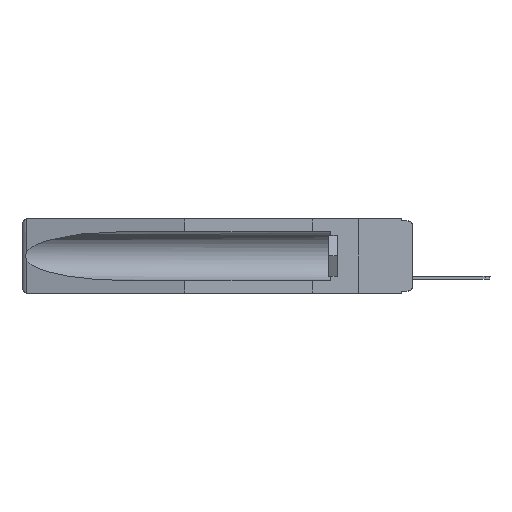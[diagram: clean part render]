
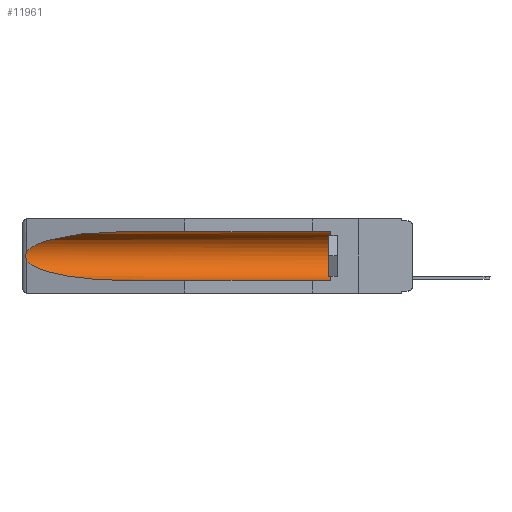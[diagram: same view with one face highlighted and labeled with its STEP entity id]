
A CAD part, left-side view. The second image highlights one B-rep face of the part: STEP entity #11961.
In plain terms, the highlighted cylindrical face has radius 2.857 mm (diameter 5.715 mm), a partial arc.
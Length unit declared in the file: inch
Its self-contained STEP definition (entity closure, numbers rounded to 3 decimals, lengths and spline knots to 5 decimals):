
#261 = DIRECTION ( 'NONE',  ( 0., -1., 0. ) ) ;
#290 = ORIENTED_EDGE ( 'NONE', *, *, #14992, .T. ) ;
#526 = CARTESIAN_POINT ( 'NONE',  ( 0.2673, 1.5327, -0.16383 ) ) ;
#824 = CARTESIAN_POINT ( 'NONE',  ( 0.155, 1.07973, -0.059 ) ) ;
#921 = CARTESIAN_POINT ( 'NONE',  ( 0.26597, 1.5296, -0.19026 ) ) ;
#1210 = CARTESIAN_POINT ( 'NONE',  ( 0.26537, 1.52718, -0.19328 ) ) ;
#1668 = CARTESIAN_POINT ( 'NONE',  ( 0.26537, 1.52718, -0.14972 ) ) ;
#1896 = CARTESIAN_POINT ( 'NONE',  ( 0.2675, 1.53308, -0.17534 ) ) ;
#1996 = VERTEX_POINT ( 'NONE', #824 ) ;
#2424 = CARTESIAN_POINT ( 'NONE',  ( 0.26537, 1.52718, -0.19328 ) ) ;
#3214 = CARTESIAN_POINT ( 'NONE',  ( 0.25451, 1.48313, -0.09465 ) ) ;
#3431 = LINE ( 'NONE', #4600, #3913 ) ;
#3781 = CARTESIAN_POINT ( 'NONE',  ( 0.2673, 1.53269, -0.17917 ) ) ;
#3913 = VECTOR ( 'NONE', #6248, 39.37008 ) ;
#4562 = CARTESIAN_POINT ( 'NONE',  ( 0.155, 0.126, -0.059 ) ) ;
#4600 = CARTESIAN_POINT ( 'NONE',  ( 0.155, -0.30754, -0.059 ) ) ;
#4889 = CARTESIAN_POINT ( 'NONE',  ( 0.155, 0.126, -0.284 ) ) ;
#4952 = DIRECTION ( 'NONE',  ( 0., 0., 1. ) ) ;
#5081 = CARTESIAN_POINT ( 'NONE',  ( 0.155, -0.30754, -0.284 ) ) ;
#5817 = ORIENTED_EDGE ( 'NONE', *, *, #17352, .T. ) ;
#5830 = CARTESIAN_POINT ( 'NONE',  ( 0.21114, 1.30732, -0.284 ) ) ;
#6248 = DIRECTION ( 'NONE',  ( 0., 1., 0. ) ) ;
#6476 = CARTESIAN_POINT ( 'NONE',  ( 0.155, 1.07973, -0.284 ) ) ;
#6992 = ORIENTED_EDGE ( 'NONE', *, *, #13037, .T. ) ;
#7486 = VECTOR ( 'NONE', #17554, 39.37008 ) ;
#7591 = B_SPLINE_CURVE_WITH_KNOTS ( 'NONE', 3,
 ( #15887, #8298, #17680, #526, #14537, #1896, #3781, #11750, #921, #2424 ),
 .UNSPECIFIED., .F., .F.,
 ( 4, 2, 2, 2, 4 ),
 ( 0., 0.00029, 0.00058, 0.00087, 0.00117 ),
 .UNSPECIFIED. ) ;
#7593 = CARTESIAN_POINT ( 'NONE',  ( 0.155, 1.07973, -0.284 ) ) ;
#8298 = CARTESIAN_POINT ( 'NONE',  ( 0.26597, 1.52961, -0.15275 ) ) ;
#8745 = FACE_OUTER_BOUND ( 'NONE', #11232, .T. ) ;
#8973 = LINE ( 'NONE', #5081, #7486 ) ;
#9035 = ORIENTED_EDGE ( 'NONE', *, *, #14960, .F. ) ;
#9303 = VERTEX_POINT ( 'NONE', #6476 ) ;
#9597 = CARTESIAN_POINT ( 'NONE',  ( 0.155, 0.126, -0.1715 ) ) ;
#9755 = CARTESIAN_POINT ( 'NONE',  ( 0.26537, 1.52718, -0.14972 ) ) ;
#9760 = ORIENTED_EDGE ( 'NONE', *, *, #15395, .T. ) ;
#9935 = EDGE_CURVE ( 'NONE', #19535, #9303, #16304, .T. ) ;
#10086 = VERTEX_POINT ( 'NONE', #4889 ) ;
#10410 = DIRECTION ( 'NONE',  ( 0., 1., 0. ) ) ;
#10870 = ORIENTED_EDGE ( 'NONE', *, *, #9935, .T. ) ;
#11232 = EDGE_LOOP ( 'NONE', ( #9760, #290, #10870, #9035, #6992, #5817 ) ) ;
#11750 = CARTESIAN_POINT ( 'NONE',  ( 0.26655, 1.53094, -0.18657 ) ) ;
#11961 = ADVANCED_FACE ( 'NONE', ( #8745 ), #18419, .F. ) ;
#12300 = CARTESIAN_POINT ( 'NONE',  ( 0.25451, 1.48313, -0.24835 ) ) ;
#12471 =( BOUNDED_CURVE ( )  B_SPLINE_CURVE ( 3, ( #13891, #20075, #3214, #1668 ),
 .UNSPECIFIED., .F., .T. ) 
 B_SPLINE_CURVE_WITH_KNOTS ( ( 4, 4 ),
 ( 4.71239, 6.08839 ),
 .UNSPECIFIED. ) 
 CURVE ( )  GEOMETRIC_REPRESENTATION_ITEM ( )  RATIONAL_B_SPLINE_CURVE ( ( 1., 0.848, 0.848, 1. ) ) 
 REPRESENTATION_ITEM ( '' )  );
#13037 = EDGE_CURVE ( 'NONE', #10086, #19279, #15030, .T. ) ;
#13251 = DIRECTION ( 'NONE',  ( 0., 0., 1. ) ) ;
#13891 = CARTESIAN_POINT ( 'NONE',  ( 0.155, 1.07973, -0.059 ) ) ;
#14537 = CARTESIAN_POINT ( 'NONE',  ( 0.2675, 1.53308, -0.16763 ) ) ;
#14960 = EDGE_CURVE ( 'NONE', #10086, #9303, #8973, .T. ) ;
#14992 = EDGE_CURVE ( 'NONE', #17053, #19535, #7591, .T. ) ;
#15030 = CIRCLE ( 'NONE', #15631, 0.1125 ) ;
#15395 = EDGE_CURVE ( 'NONE', #1996, #17053, #12471, .T. ) ;
#15631 = AXIS2_PLACEMENT_3D ( 'NONE', #9597, #261, #4952 ) ;
#15887 = CARTESIAN_POINT ( 'NONE',  ( 0.26537, 1.52718, -0.14972 ) ) ;
#16176 = CARTESIAN_POINT ( 'NONE',  ( 0.26537, 1.52718, -0.19328 ) ) ;
#16304 =( BOUNDED_CURVE ( )  B_SPLINE_CURVE ( 3, ( #1210, #12300, #5830, #7593 ),
 .UNSPECIFIED., .F., .F. ) 
 B_SPLINE_CURVE_WITH_KNOTS ( ( 4, 4 ),
 ( 0.1948, 1.5708 ),
 .UNSPECIFIED. ) 
 CURVE ( )  GEOMETRIC_REPRESENTATION_ITEM ( )  RATIONAL_B_SPLINE_CURVE ( ( 1., 0.848, 0.848, 1. ) ) 
 REPRESENTATION_ITEM ( '' )  );
#16385 = AXIS2_PLACEMENT_3D ( 'NONE', #17897, #10410, #13251 ) ;
#17053 = VERTEX_POINT ( 'NONE', #9755 ) ;
#17352 = EDGE_CURVE ( 'NONE', #19279, #1996, #3431, .T. ) ;
#17554 = DIRECTION ( 'NONE',  ( 0., 1., 0. ) ) ;
#17680 = CARTESIAN_POINT ( 'NONE',  ( 0.26654, 1.53092, -0.15636 ) ) ;
#17897 = CARTESIAN_POINT ( 'NONE',  ( 0.155, -0.30754, -0.1715 ) ) ;
#18419 = CYLINDRICAL_SURFACE ( 'NONE', #16385, 0.1125 ) ;
#19279 = VERTEX_POINT ( 'NONE', #4562 ) ;
#19535 = VERTEX_POINT ( 'NONE', #16176 ) ;
#20075 = CARTESIAN_POINT ( 'NONE',  ( 0.21114, 1.30732, -0.059 ) ) ;
